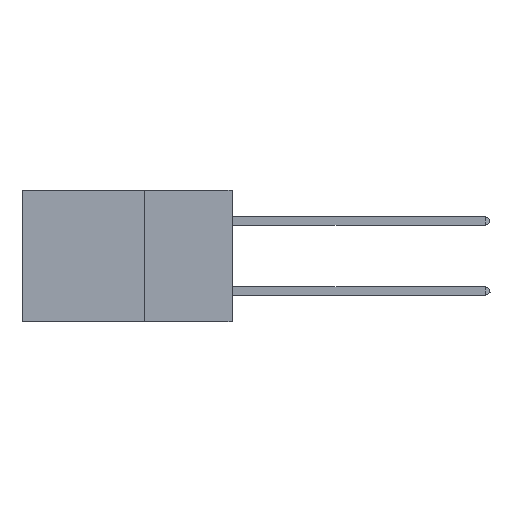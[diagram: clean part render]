
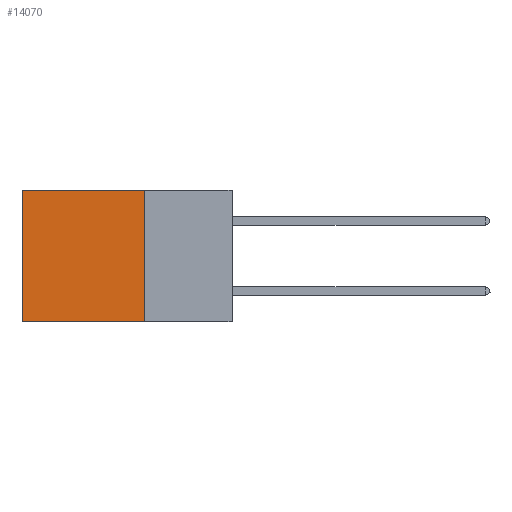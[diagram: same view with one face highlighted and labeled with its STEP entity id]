
A CAD part, left-side view. The second image highlights one B-rep face of the part: STEP entity #14070.
In plain terms, the highlighted planar face has unit normal (-1, 0, 0).
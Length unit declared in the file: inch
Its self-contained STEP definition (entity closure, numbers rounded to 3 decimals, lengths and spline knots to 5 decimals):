
#837 = VERTEX_POINT ( 'NONE', #11978 ) ;
#1214 = AXIS2_PLACEMENT_3D ( 'NONE', #8909, #8784, #5772 ) ;
#2119 = FACE_OUTER_BOUND ( 'NONE', #12200, .T. ) ;
#2172 = CARTESIAN_POINT ( 'NONE',  ( 0.2875, 0.25, -0.375 ) ) ;
#2610 = EDGE_CURVE ( 'NONE', #3758, #3699, #7136, .T. ) ;
#3013 = CARTESIAN_POINT ( 'NONE',  ( 0.2875, 0.25, -0.375 ) ) ;
#3579 = VECTOR ( 'NONE', #7104, 39.37008 ) ;
#3699 = VERTEX_POINT ( 'NONE', #19267 ) ;
#3707 = LINE ( 'NONE', #18420, #13229 ) ;
#3758 = VERTEX_POINT ( 'NONE', #7565 ) ;
#4097 = VERTEX_POINT ( 'NONE', #2172 ) ;
#5772 = DIRECTION ( 'NONE',  ( 0., 0., -1. ) ) ;
#6405 = VECTOR ( 'NONE', #15187, 39.37008 ) ;
#7059 = CARTESIAN_POINT ( 'NONE',  ( 0.2875, 0.6, -0.375 ) ) ;
#7104 = DIRECTION ( 'NONE',  ( 0., 1., 0. ) ) ;
#7136 = LINE ( 'NONE', #19086, #3579 ) ;
#7565 = CARTESIAN_POINT ( 'NONE',  ( 0.2875, 0.25, 0. ) ) ;
#8468 = ORIENTED_EDGE ( 'NONE', *, *, #14260, .F. ) ;
#8710 = PLANE ( 'NONE',  #1214 ) ;
#8724 = VECTOR ( 'NONE', #11750, 39.37008 ) ;
#8784 = DIRECTION ( 'NONE',  ( 1., 0., 0. ) ) ;
#8909 = CARTESIAN_POINT ( 'NONE',  ( 0.2875, 0.25, -0.375 ) ) ;
#9159 = EDGE_CURVE ( 'NONE', #4097, #837, #3707, .T. ) ;
#9983 = ORIENTED_EDGE ( 'NONE', *, *, #2610, .T. ) ;
#10469 = LINE ( 'NONE', #3013, #6405 ) ;
#10541 = ORIENTED_EDGE ( 'NONE', *, *, #19377, .T. ) ;
#11750 = DIRECTION ( 'NONE',  ( 0., 0., -1. ) ) ;
#11978 = CARTESIAN_POINT ( 'NONE',  ( 0.2875, 0.6, -0.375 ) ) ;
#12200 = EDGE_LOOP ( 'NONE', ( #10541, #15229, #8468, #9983 ) ) ;
#13229 = VECTOR ( 'NONE', #13729, 39.37008 ) ;
#13729 = DIRECTION ( 'NONE',  ( 0., 1., 0. ) ) ;
#13976 = LINE ( 'NONE', #7059, #8724 ) ;
#14070 = ADVANCED_FACE ( 'NONE', ( #2119 ), #8710, .F. ) ;
#14260 = EDGE_CURVE ( 'NONE', #3758, #4097, #10469, .T. ) ;
#15187 = DIRECTION ( 'NONE',  ( 0., 0., -1. ) ) ;
#15229 = ORIENTED_EDGE ( 'NONE', *, *, #9159, .F. ) ;
#18420 = CARTESIAN_POINT ( 'NONE',  ( 0.2875, 0.25, -0.375 ) ) ;
#19086 = CARTESIAN_POINT ( 'NONE',  ( 0.2875, 0.25, 0. ) ) ;
#19267 = CARTESIAN_POINT ( 'NONE',  ( 0.2875, 0.6, 0. ) ) ;
#19377 = EDGE_CURVE ( 'NONE', #3699, #837, #13976, .T. ) ;
